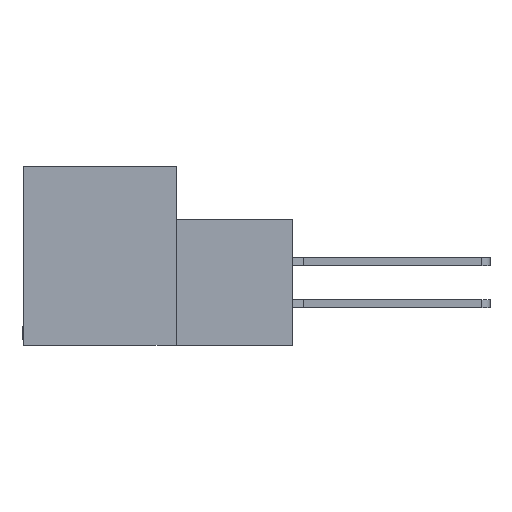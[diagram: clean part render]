
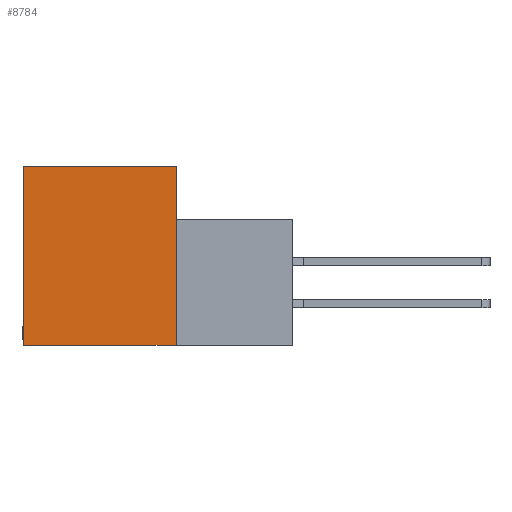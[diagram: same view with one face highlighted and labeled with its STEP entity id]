
A CAD part, left-side view. The second image highlights one B-rep face of the part: STEP entity #8784.
In plain terms, the highlighted planar face has unit normal (-1, 0, 0).
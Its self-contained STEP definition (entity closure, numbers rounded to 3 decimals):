
#1019 = CARTESIAN_POINT ( 'NONE',  ( 0., 0., 0. ) ) ;
#1226 = EDGE_CURVE ( 'NONE', #4548, #11344, #15988, .T. ) ;
#1493 = DIRECTION ( 'NONE',  ( 0., -1., 0. ) ) ;
#1567 = CARTESIAN_POINT ( 'NONE',  ( 0., 11.506, 0. ) ) ;
#3042 = DIRECTION ( 'NONE',  ( 0., 1., 0. ) ) ;
#3746 = VECTOR ( 'NONE', #5435, 1000. ) ;
#4400 = CARTESIAN_POINT ( 'NONE',  ( 0., 0., -13.487 ) ) ;
#4548 = VERTEX_POINT ( 'NONE', #4908 ) ;
#4800 = CARTESIAN_POINT ( 'NONE',  ( 0., 11.506, -13.487 ) ) ;
#4908 = CARTESIAN_POINT ( 'NONE',  ( 0., 11.506, -13.487 ) ) ;
#5418 = ORIENTED_EDGE ( 'NONE', *, *, #6033, .F. ) ;
#5435 = DIRECTION ( 'NONE',  ( 0., 0., -1. ) ) ;
#6033 = EDGE_CURVE ( 'NONE', #23831, #4548, #17308, .T. ) ;
#6965 = DIRECTION ( 'NONE',  ( 0., 0., 1. ) ) ;
#7781 = VERTEX_POINT ( 'NONE', #21054 ) ;
#8110 = EDGE_LOOP ( 'NONE', ( #5418, #13916, #14399, #12517 ) ) ;
#8680 = DIRECTION ( 'NONE',  ( 0., 0., -1. ) ) ;
#8784 = ADVANCED_FACE ( 'NONE', ( #19782 ), #23062, .F. ) ;
#9285 = CARTESIAN_POINT ( 'NONE',  ( 0., 11.506, 0. ) ) ;
#11238 = EDGE_CURVE ( 'NONE', #11344, #7781, #17072, .T. ) ;
#11344 = VERTEX_POINT ( 'NONE', #9285 ) ;
#12517 = ORIENTED_EDGE ( 'NONE', *, *, #1226, .F. ) ;
#13916 = ORIENTED_EDGE ( 'NONE', *, *, #18525, .F. ) ;
#13948 = CARTESIAN_POINT ( 'NONE',  ( 0., -8.814, -13.487 ) ) ;
#14399 = ORIENTED_EDGE ( 'NONE', *, *, #11238, .F. ) ;
#14501 = AXIS2_PLACEMENT_3D ( 'NONE', #1019, #17820, #8680 ) ;
#15415 = VECTOR ( 'NONE', #6965, 1000. ) ;
#15988 = LINE ( 'NONE', #4800, #15415 ) ;
#17072 = LINE ( 'NONE', #1567, #22844 ) ;
#17245 = LINE ( 'NONE', #18373, #3746 ) ;
#17308 = LINE ( 'NONE', #13948, #23075 ) ;
#17820 = DIRECTION ( 'NONE',  ( 1., 0., 0. ) ) ;
#18373 = CARTESIAN_POINT ( 'NONE',  ( 0., 0., 0. ) ) ;
#18525 = EDGE_CURVE ( 'NONE', #7781, #23831, #17245, .T. ) ;
#19782 = FACE_OUTER_BOUND ( 'NONE', #8110, .T. ) ;
#21054 = CARTESIAN_POINT ( 'NONE',  ( 0., 0., 0. ) ) ;
#22844 = VECTOR ( 'NONE', #1493, 1000. ) ;
#23062 = PLANE ( 'NONE',  #14501 ) ;
#23075 = VECTOR ( 'NONE', #3042, 1000. ) ;
#23831 = VERTEX_POINT ( 'NONE', #4400 ) ;
